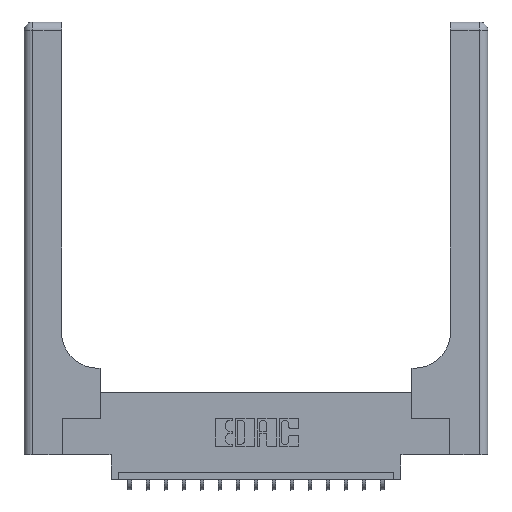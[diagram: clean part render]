
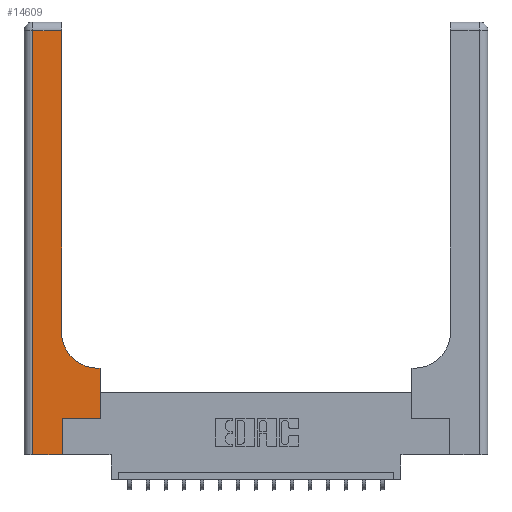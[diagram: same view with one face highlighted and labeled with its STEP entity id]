
A CAD part, top view. The second image highlights one B-rep face of the part: STEP entity #14609.
In plain terms, the highlighted planar face has unit normal (0, 0, 1).
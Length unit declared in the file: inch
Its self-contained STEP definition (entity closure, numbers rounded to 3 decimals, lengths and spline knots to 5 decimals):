
#92 = CIRCLE ( 'NONE', #14396, 0.25 ) ;
#362 = ORIENTED_EDGE ( 'NONE', *, *, #8829, .T. ) ;
#370 = VERTEX_POINT ( 'NONE', #7920 ) ;
#678 = ORIENTED_EDGE ( 'NONE', *, *, #4564, .T. ) ;
#1156 = CARTESIAN_POINT ( 'NONE',  ( 0., 2.94, 0.37 ) ) ;
#1349 = VECTOR ( 'NONE', #9822, 39.37008 ) ;
#2292 = CARTESIAN_POINT ( 'NONE',  ( 0., 0., 0.37 ) ) ;
#2366 = VECTOR ( 'NONE', #13703, 39.37008 ) ;
#2639 = CARTESIAN_POINT ( 'NONE',  ( 0.265, 0., 0.37 ) ) ;
#3218 = DIRECTION ( 'NONE',  ( 1., 0., 0. ) ) ;
#3269 = LINE ( 'NONE', #2292, #2366 ) ;
#3308 = PLANE ( 'NONE',  #16794 ) ;
#4259 = VERTEX_POINT ( 'NONE', #12736 ) ;
#4471 = LINE ( 'NONE', #17193, #7929 ) ;
#4564 = EDGE_CURVE ( 'NONE', #4259, #5848, #3269, .T. ) ;
#4773 = DIRECTION ( 'NONE',  ( -1., 0., 0. ) ) ;
#4966 = VECTOR ( 'NONE', #10779, 39.37008 ) ;
#5006 = CARTESIAN_POINT ( 'NONE',  ( 0.265, 0., 0.37 ) ) ;
#5516 = CARTESIAN_POINT ( 'NONE',  ( 0.26, 2.94, 0.37 ) ) ;
#5713 = CARTESIAN_POINT ( 'NONE',  ( 0.26, 0.6, 0.37 ) ) ;
#5820 = CARTESIAN_POINT ( 'NONE',  ( 0.528, 0.25, 0.37 ) ) ;
#5848 = VERTEX_POINT ( 'NONE', #2639 ) ;
#6067 = ORIENTED_EDGE ( 'NONE', *, *, #7688, .T. ) ;
#6111 = CARTESIAN_POINT ( 'NONE',  ( 0.528, 0.6, 0.37 ) ) ;
#6816 = ORIENTED_EDGE ( 'NONE', *, *, #9675, .T. ) ;
#6824 = FACE_OUTER_BOUND ( 'NONE', #11547, .T. ) ;
#7111 = CARTESIAN_POINT ( 'NONE',  ( 0.51, 0.6, 0.37 ) ) ;
#7524 = ORIENTED_EDGE ( 'NONE', *, *, #16292, .T. ) ;
#7658 = EDGE_CURVE ( 'NONE', #17436, #16874, #8863, .T. ) ;
#7668 = CARTESIAN_POINT ( 'NONE',  ( 0., 3., 0.37 ) ) ;
#7688 = EDGE_CURVE ( 'NONE', #8832, #4259, #15360, .T. ) ;
#7920 = CARTESIAN_POINT ( 'NONE',  ( 0.265, 0.25, 0.37 ) ) ;
#7929 = VECTOR ( 'NONE', #11706, 39.37008 ) ;
#7979 = VECTOR ( 'NONE', #17785, 39.37008 ) ;
#8648 = CARTESIAN_POINT ( 'NONE',  ( 0.06, 2.94, 0.37 ) ) ;
#8711 = LINE ( 'NONE', #13019, #12848 ) ;
#8733 = DIRECTION ( 'NONE',  ( 0., 0., -1. ) ) ;
#8829 = EDGE_CURVE ( 'NONE', #16993, #17424, #15540, .T. ) ;
#8832 = VERTEX_POINT ( 'NONE', #8648 ) ;
#8863 = LINE ( 'NONE', #9216, #15801 ) ;
#9062 = LINE ( 'NONE', #1156, #1349 ) ;
#9216 = CARTESIAN_POINT ( 'NONE',  ( 0.26, 3., 0.37 ) ) ;
#9558 = VERTEX_POINT ( 'NONE', #5820 ) ;
#9647 = ORIENTED_EDGE ( 'NONE', *, *, #7658, .T. ) ;
#9675 = EDGE_CURVE ( 'NONE', #370, #9558, #4471, .T. ) ;
#9822 = DIRECTION ( 'NONE',  ( -1., 0., 0. ) ) ;
#10205 = DIRECTION ( 'NONE',  ( 0., 1., 0. ) ) ;
#10605 = DIRECTION ( 'NONE',  ( 0., 1., 0. ) ) ;
#10779 = DIRECTION ( 'NONE',  ( 0., 1., 0. ) ) ;
#11192 = EDGE_CURVE ( 'NONE', #17424, #17436, #92, .T. ) ;
#11547 = EDGE_LOOP ( 'NONE', ( #9647, #7524, #6067, #678, #13940, #6816, #14162, #362, #13262 ) ) ;
#11706 = DIRECTION ( 'NONE',  ( 1., 0., 0. ) ) ;
#11857 = VECTOR ( 'NONE', #18295, 39.37008 ) ;
#12433 = EDGE_CURVE ( 'NONE', #9558, #16993, #8711, .T. ) ;
#12736 = CARTESIAN_POINT ( 'NONE',  ( 0.06, 0., 0.37 ) ) ;
#12848 = VECTOR ( 'NONE', #10205, 39.37008 ) ;
#13019 = CARTESIAN_POINT ( 'NONE',  ( 0.528, 0.25, 0.37 ) ) ;
#13262 = ORIENTED_EDGE ( 'NONE', *, *, #11192, .T. ) ;
#13294 = DIRECTION ( 'NONE',  ( 0., 0., -1. ) ) ;
#13703 = DIRECTION ( 'NONE',  ( 1., 0., 0. ) ) ;
#13735 = CARTESIAN_POINT ( 'NONE',  ( 0.06, 3., 0.37 ) ) ;
#13940 = ORIENTED_EDGE ( 'NONE', *, *, #14756, .T. ) ;
#14162 = ORIENTED_EDGE ( 'NONE', *, *, #12433, .T. ) ;
#14396 = AXIS2_PLACEMENT_3D ( 'NONE', #17005, #8733, #3218 ) ;
#14609 = ADVANCED_FACE ( 'NONE', ( #6824 ), #3308, .F. ) ;
#14756 = EDGE_CURVE ( 'NONE', #5848, #370, #15787, .T. ) ;
#15360 = LINE ( 'NONE', #13735, #7979 ) ;
#15537 = CARTESIAN_POINT ( 'NONE',  ( 0.26, 0.85, 0.37 ) ) ;
#15540 = LINE ( 'NONE', #5713, #11857 ) ;
#15787 = LINE ( 'NONE', #5006, #4966 ) ;
#15801 = VECTOR ( 'NONE', #10605, 39.37008 ) ;
#16292 = EDGE_CURVE ( 'NONE', #16874, #8832, #9062, .T. ) ;
#16794 = AXIS2_PLACEMENT_3D ( 'NONE', #7668, #13294, #4773 ) ;
#16874 = VERTEX_POINT ( 'NONE', #5516 ) ;
#16993 = VERTEX_POINT ( 'NONE', #6111 ) ;
#17005 = CARTESIAN_POINT ( 'NONE',  ( 0.51, 0.85, 0.37 ) ) ;
#17193 = CARTESIAN_POINT ( 'NONE',  ( 0.265, 0.25, 0.37 ) ) ;
#17424 = VERTEX_POINT ( 'NONE', #7111 ) ;
#17436 = VERTEX_POINT ( 'NONE', #15537 ) ;
#17785 = DIRECTION ( 'NONE',  ( 0., -1., 0. ) ) ;
#18295 = DIRECTION ( 'NONE',  ( -1., 0., 0. ) ) ;
